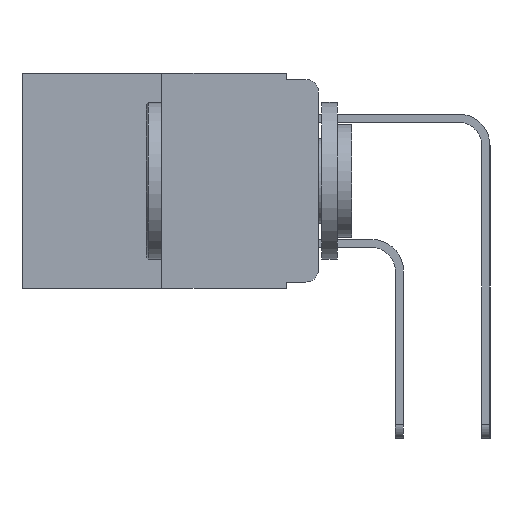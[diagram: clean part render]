
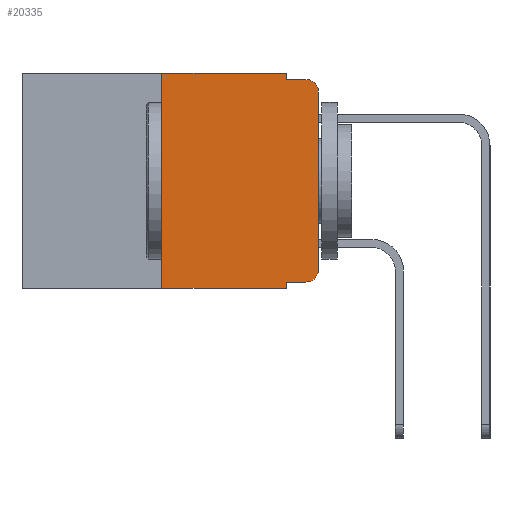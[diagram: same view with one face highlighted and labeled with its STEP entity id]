
A CAD part, left-side view. The second image highlights one B-rep face of the part: STEP entity #20335.
In plain terms, the highlighted planar face has unit normal (-1, 0, 0).
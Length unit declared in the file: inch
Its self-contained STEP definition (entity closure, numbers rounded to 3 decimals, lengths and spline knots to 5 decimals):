
#74 = VERTEX_POINT ( 'NONE', #17093 ) ;
#395 = DIRECTION ( 'NONE',  ( 0., 0., -1. ) ) ;
#1013 = LINE ( 'NONE', #25309, #5984 ) ;
#1157 = VERTEX_POINT ( 'NONE', #11425 ) ;
#1309 = VECTOR ( 'NONE', #25371, 39.37008 ) ;
#1539 = VECTOR ( 'NONE', #21054, 39.37008 ) ;
#1623 = ORIENTED_EDGE ( 'NONE', *, *, #20298, .T. ) ;
#1909 = VECTOR ( 'NONE', #19449, 39.37008 ) ;
#2786 = EDGE_CURVE ( 'NONE', #5199, #21236, #20271, .T. ) ;
#2915 = ORIENTED_EDGE ( 'NONE', *, *, #25097, .T. ) ;
#3672 = VERTEX_POINT ( 'NONE', #21106 ) ;
#4206 = EDGE_CURVE ( 'NONE', #13411, #5033, #18191, .T. ) ;
#4552 = ORIENTED_EDGE ( 'NONE', *, *, #4206, .F. ) ;
#4950 = EDGE_CURVE ( 'NONE', #21236, #13411, #22359, .T. ) ;
#5033 = VERTEX_POINT ( 'NONE', #14219 ) ;
#5078 = PLANE ( 'NONE',  #22358 ) ;
#5199 = VERTEX_POINT ( 'NONE', #5426 ) ;
#5426 = CARTESIAN_POINT ( 'NONE',  ( 0., 0.25, -0.343 ) ) ;
#5651 = EDGE_CURVE ( 'NONE', #5033, #13043, #19682, .T. ) ;
#5984 = VECTOR ( 'NONE', #19602, 39.37008 ) ;
#6932 = LINE ( 'NONE', #11490, #1309 ) ;
#7066 = EDGE_CURVE ( 'NONE', #3672, #13043, #12923, .T. ) ;
#7225 = DIRECTION ( 'NONE',  ( 0., 0., -1. ) ) ;
#7445 = CARTESIAN_POINT ( 'NONE',  ( 0., 0.02, -0.01 ) ) ;
#7539 = LINE ( 'NONE', #21285, #1909 ) ;
#8486 = EDGE_CURVE ( 'NONE', #74, #3672, #1013, .T. ) ;
#8507 = DIRECTION ( 'NONE',  ( -1., 0., 0. ) ) ;
#10658 = LINE ( 'NONE', #24829, #18987 ) ;
#10798 = CARTESIAN_POINT ( 'NONE',  ( 0., 0.051, 0. ) ) ;
#11425 = CARTESIAN_POINT ( 'NONE',  ( 0., 0.051, -0.343 ) ) ;
#11490 = CARTESIAN_POINT ( 'NONE',  ( 0., 0.051, 0. ) ) ;
#11516 = ORIENTED_EDGE ( 'NONE', *, *, #4950, .F. ) ;
#11719 = CARTESIAN_POINT ( 'NONE',  ( 0., 0.25, 0. ) ) ;
#12258 = VERTEX_POINT ( 'NONE', #14437 ) ;
#12598 = CARTESIAN_POINT ( 'NONE',  ( 0., 0.051, -0.333 ) ) ;
#12923 = CIRCLE ( 'NONE', #13112, 0.02 ) ;
#12999 = DIRECTION ( 'NONE',  ( -1., 0., 0. ) ) ;
#13043 = VERTEX_POINT ( 'NONE', #7445 ) ;
#13101 = ORIENTED_EDGE ( 'NONE', *, *, #8486, .T. ) ;
#13112 = AXIS2_PLACEMENT_3D ( 'NONE', #24855, #12999, #395 ) ;
#13411 = VERTEX_POINT ( 'NONE', #10798 ) ;
#13680 = VECTOR ( 'NONE', #17498, 39.37008 ) ;
#14014 = EDGE_LOOP ( 'NONE', ( #13101, #23673, #19158, #4552, #11516, #22160, #1623, #18871, #2915, #14135 ) ) ;
#14045 = AXIS2_PLACEMENT_3D ( 'NONE', #20706, #8507, #22612 ) ;
#14135 = ORIENTED_EDGE ( 'NONE', *, *, #23819, .T. ) ;
#14219 = CARTESIAN_POINT ( 'NONE',  ( 0., 0.051, -0.01 ) ) ;
#14437 = CARTESIAN_POINT ( 'NONE',  ( 0., 0.02, -0.333 ) ) ;
#15802 = VERTEX_POINT ( 'NONE', #12598 ) ;
#16973 = CARTESIAN_POINT ( 'NONE',  ( 0., 0.051, 0. ) ) ;
#17093 = CARTESIAN_POINT ( 'NONE',  ( 0., 0., -0.313 ) ) ;
#17399 = CARTESIAN_POINT ( 'NONE',  ( 0., 0.051, -0.01 ) ) ;
#17498 = DIRECTION ( 'NONE',  ( 0., -1., 0. ) ) ;
#17833 = VECTOR ( 'NONE', #25974, 39.37008 ) ;
#17904 = FACE_OUTER_BOUND ( 'NONE', #14014, .T. ) ;
#18119 = CIRCLE ( 'NONE', #14045, 0.02 ) ;
#18191 = LINE ( 'NONE', #16973, #1539 ) ;
#18871 = ORIENTED_EDGE ( 'NONE', *, *, #21077, .F. ) ;
#18987 = VECTOR ( 'NONE', #22887, 39.37008 ) ;
#19158 = ORIENTED_EDGE ( 'NONE', *, *, #5651, .F. ) ;
#19449 = DIRECTION ( 'NONE',  ( 0., -1., 0. ) ) ;
#19534 = DIRECTION ( 'NONE',  ( 1., 0., 0. ) ) ;
#19602 = DIRECTION ( 'NONE',  ( 0., 0., 1. ) ) ;
#19682 = LINE ( 'NONE', #17399, #13680 ) ;
#20271 = LINE ( 'NONE', #21259, #22053 ) ;
#20298 = EDGE_CURVE ( 'NONE', #5199, #1157, #7539, .T. ) ;
#20335 = ADVANCED_FACE ( 'NONE', ( #17904 ), #5078, .F. ) ;
#20706 = CARTESIAN_POINT ( 'NONE',  ( 0., 0.02, -0.313 ) ) ;
#21054 = DIRECTION ( 'NONE',  ( 0., 0., -1. ) ) ;
#21077 = EDGE_CURVE ( 'NONE', #15802, #1157, #6932, .T. ) ;
#21106 = CARTESIAN_POINT ( 'NONE',  ( 0., 0., -0.03 ) ) ;
#21236 = VERTEX_POINT ( 'NONE', #11719 ) ;
#21259 = CARTESIAN_POINT ( 'NONE',  ( 0., 0.25, 0. ) ) ;
#21285 = CARTESIAN_POINT ( 'NONE',  ( 0., 0.473, -0.343 ) ) ;
#21623 = DIRECTION ( 'NONE',  ( 0., 0., 1. ) ) ;
#22053 = VECTOR ( 'NONE', #21623, 39.37008 ) ;
#22160 = ORIENTED_EDGE ( 'NONE', *, *, #2786, .F. ) ;
#22358 = AXIS2_PLACEMENT_3D ( 'NONE', #23315, #19534, #7225 ) ;
#22359 = LINE ( 'NONE', #26008, #17833 ) ;
#22612 = DIRECTION ( 'NONE',  ( 0., 0., -1. ) ) ;
#22887 = DIRECTION ( 'NONE',  ( 0., -1., 0. ) ) ;
#23315 = CARTESIAN_POINT ( 'NONE',  ( 0., 0.473, 0. ) ) ;
#23673 = ORIENTED_EDGE ( 'NONE', *, *, #7066, .T. ) ;
#23819 = EDGE_CURVE ( 'NONE', #12258, #74, #18119, .T. ) ;
#24829 = CARTESIAN_POINT ( 'NONE',  ( 0., 0.051, -0.333 ) ) ;
#24855 = CARTESIAN_POINT ( 'NONE',  ( 0., 0.02, -0.03 ) ) ;
#25097 = EDGE_CURVE ( 'NONE', #15802, #12258, #10658, .T. ) ;
#25309 = CARTESIAN_POINT ( 'NONE',  ( 0., 0., 0. ) ) ;
#25371 = DIRECTION ( 'NONE',  ( 0., 0., -1. ) ) ;
#25974 = DIRECTION ( 'NONE',  ( 0., -1., 0. ) ) ;
#26008 = CARTESIAN_POINT ( 'NONE',  ( 0., 0.473, 0. ) ) ;
